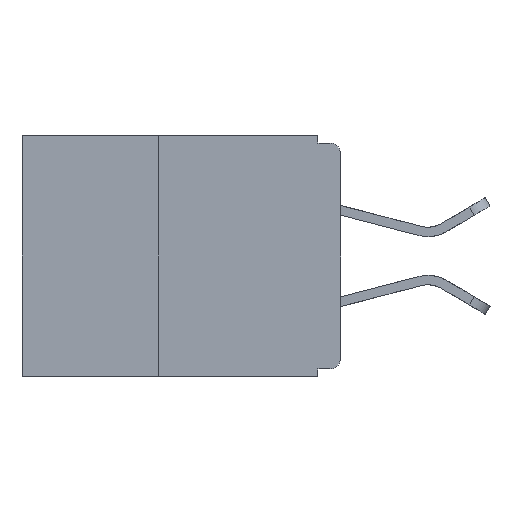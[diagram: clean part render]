
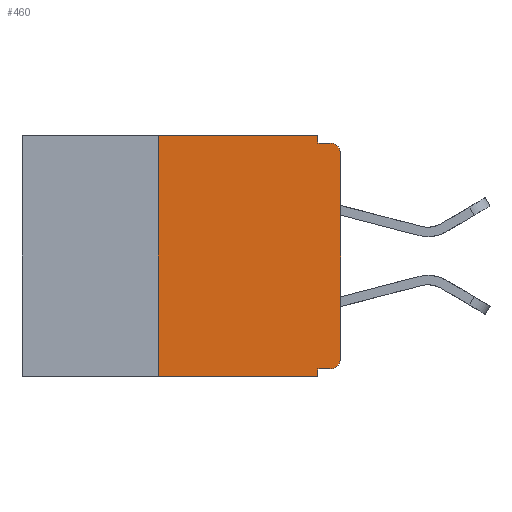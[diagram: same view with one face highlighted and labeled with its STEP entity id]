
A CAD part, left-side view. The second image highlights one B-rep face of the part: STEP entity #460.
In plain terms, the highlighted planar face has unit normal (-1, 0, 0).
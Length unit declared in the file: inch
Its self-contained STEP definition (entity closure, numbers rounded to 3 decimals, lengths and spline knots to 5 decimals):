
#223 = DIRECTION ( 'NONE',  ( 0., 0., -1. ) ) ;
#285 = EDGE_CURVE ( 'NONE', #17375, #4428, #4743, .T. ) ;
#400 = EDGE_CURVE ( 'NONE', #8476, #15993, #18680, .T. ) ;
#460 = ADVANCED_FACE ( 'NONE', ( #1088 ), #10878, .F. ) ;
#977 = CARTESIAN_POINT ( 'NONE',  ( 0., 0.031, 0. ) ) ;
#1088 = FACE_OUTER_BOUND ( 'NONE', #18383, .T. ) ;
#1360 = ORIENTED_EDGE ( 'NONE', *, *, #400, .F. ) ;
#1376 = ORIENTED_EDGE ( 'NONE', *, *, #17903, .F. ) ;
#2164 = CARTESIAN_POINT ( 'NONE',  ( 0., 0.015, -0.01 ) ) ;
#2228 = CARTESIAN_POINT ( 'NONE',  ( 0., 0., 0. ) ) ;
#2318 = DIRECTION ( 'NONE',  ( 0., -1., 0. ) ) ;
#2415 = CARTESIAN_POINT ( 'NONE',  ( 0., 0.437, 0. ) ) ;
#2435 = VERTEX_POINT ( 'NONE', #8285 ) ;
#3471 = AXIS2_PLACEMENT_3D ( 'NONE', #15699, #6561, #17208 ) ;
#3631 = CIRCLE ( 'NONE', #3471, 0.015 ) ;
#3760 = DIRECTION ( 'NONE',  ( 0., 0., -1. ) ) ;
#4344 = VECTOR ( 'NONE', #7113, 39.37008 ) ;
#4399 = LINE ( 'NONE', #14602, #10470 ) ;
#4428 = VERTEX_POINT ( 'NONE', #18686 ) ;
#4743 = LINE ( 'NONE', #12650, #12577 ) ;
#5002 = ORIENTED_EDGE ( 'NONE', *, *, #285, .F. ) ;
#6561 = DIRECTION ( 'NONE',  ( -1., 0., 0. ) ) ;
#6858 = AXIS2_PLACEMENT_3D ( 'NONE', #18980, #9917, #223 ) ;
#7113 = DIRECTION ( 'NONE',  ( 0., 1., 0. ) ) ;
#7298 = VECTOR ( 'NONE', #2318, 39.37008 ) ;
#7758 = VERTEX_POINT ( 'NONE', #977 ) ;
#7860 = CARTESIAN_POINT ( 'NONE',  ( 0., 0.25, 0. ) ) ;
#7988 = LINE ( 'NONE', #19134, #11572 ) ;
#8125 = LINE ( 'NONE', #2228, #15703 ) ;
#8285 = CARTESIAN_POINT ( 'NONE',  ( 0., 0., -0.305 ) ) ;
#8476 = VERTEX_POINT ( 'NONE', #13540 ) ;
#8479 = ORIENTED_EDGE ( 'NONE', *, *, #14955, .F. ) ;
#8782 = EDGE_CURVE ( 'NONE', #18211, #7758, #19862, .T. ) ;
#9809 = CARTESIAN_POINT ( 'NONE',  ( 0., 0.25, -0.33 ) ) ;
#9901 = ORIENTED_EDGE ( 'NONE', *, *, #8782, .F. ) ;
#9917 = DIRECTION ( 'NONE',  ( -1., 0., 0. ) ) ;
#10164 = CARTESIAN_POINT ( 'NONE',  ( 0., 0.25, -0.33 ) ) ;
#10266 = DIRECTION ( 'NONE',  ( 0., 0., 1. ) ) ;
#10390 = EDGE_CURVE ( 'NONE', #17261, #18211, #15106, .T. ) ;
#10470 = VECTOR ( 'NONE', #19138, 39.37008 ) ;
#10646 = VECTOR ( 'NONE', #19593, 39.37008 ) ;
#10878 = PLANE ( 'NONE',  #16770 ) ;
#11572 = VECTOR ( 'NONE', #3760, 39.37008 ) ;
#11605 = ORIENTED_EDGE ( 'NONE', *, *, #17921, .T. ) ;
#11906 = CARTESIAN_POINT ( 'NONE',  ( 0., 0.437, 0. ) ) ;
#12577 = VECTOR ( 'NONE', #15708, 39.37008 ) ;
#12650 = CARTESIAN_POINT ( 'NONE',  ( 0., 0.031, -0.33 ) ) ;
#12839 = EDGE_CURVE ( 'NONE', #15668, #2435, #18295, .T. ) ;
#13505 = CARTESIAN_POINT ( 'NONE',  ( 0., 0.031, -0.32 ) ) ;
#13540 = CARTESIAN_POINT ( 'NONE',  ( 0., 0.031, -0.01 ) ) ;
#14484 = DIRECTION ( 'NONE',  ( 1., 0., 0. ) ) ;
#14602 = CARTESIAN_POINT ( 'NONE',  ( 0., 0.437, -0.33 ) ) ;
#14638 = VECTOR ( 'NONE', #18871, 39.37008 ) ;
#14902 = DIRECTION ( 'NONE',  ( 0., 0., -1. ) ) ;
#14955 = EDGE_CURVE ( 'NONE', #7758, #8476, #7988, .T. ) ;
#15106 = LINE ( 'NONE', #9809, #14638 ) ;
#15367 = ORIENTED_EDGE ( 'NONE', *, *, #15965, .T. ) ;
#15597 = ORIENTED_EDGE ( 'NONE', *, *, #10390, .F. ) ;
#15668 = VERTEX_POINT ( 'NONE', #18117 ) ;
#15699 = CARTESIAN_POINT ( 'NONE',  ( 0., 0.015, -0.025 ) ) ;
#15703 = VECTOR ( 'NONE', #10266, 39.37008 ) ;
#15708 = DIRECTION ( 'NONE',  ( 0., 0., -1. ) ) ;
#15795 = EDGE_CURVE ( 'NONE', #18207, #15993, #3631, .T. ) ;
#15965 = EDGE_CURVE ( 'NONE', #17261, #4428, #4399, .T. ) ;
#15993 = VERTEX_POINT ( 'NONE', #2164 ) ;
#16525 = ORIENTED_EDGE ( 'NONE', *, *, #15795, .T. ) ;
#16770 = AXIS2_PLACEMENT_3D ( 'NONE', #11906, #14484, #14902 ) ;
#16918 = CARTESIAN_POINT ( 'NONE',  ( 0., 0., -0.025 ) ) ;
#17208 = DIRECTION ( 'NONE',  ( 0., 0., -1. ) ) ;
#17261 = VERTEX_POINT ( 'NONE', #10164 ) ;
#17375 = VERTEX_POINT ( 'NONE', #13505 ) ;
#17903 = EDGE_CURVE ( 'NONE', #15668, #17375, #20160, .T. ) ;
#17921 = EDGE_CURVE ( 'NONE', #2435, #18207, #8125, .T. ) ;
#18117 = CARTESIAN_POINT ( 'NONE',  ( 0., 0.015, -0.32 ) ) ;
#18207 = VERTEX_POINT ( 'NONE', #16918 ) ;
#18211 = VERTEX_POINT ( 'NONE', #7860 ) ;
#18295 = CIRCLE ( 'NONE', #6858, 0.015 ) ;
#18299 = CARTESIAN_POINT ( 'NONE',  ( 0., 0., -0.01 ) ) ;
#18383 = EDGE_LOOP ( 'NONE', ( #11605, #16525, #1360, #8479, #9901, #15597, #15367, #5002, #1376, #18735 ) ) ;
#18680 = LINE ( 'NONE', #18299, #10646 ) ;
#18686 = CARTESIAN_POINT ( 'NONE',  ( 0., 0.031, -0.33 ) ) ;
#18735 = ORIENTED_EDGE ( 'NONE', *, *, #12839, .T. ) ;
#18871 = DIRECTION ( 'NONE',  ( 0., 0., 1. ) ) ;
#18980 = CARTESIAN_POINT ( 'NONE',  ( 0., 0.015, -0.305 ) ) ;
#19134 = CARTESIAN_POINT ( 'NONE',  ( 0., 0.031, 0. ) ) ;
#19138 = DIRECTION ( 'NONE',  ( 0., -1., 0. ) ) ;
#19269 = CARTESIAN_POINT ( 'NONE',  ( 0., 0., -0.32 ) ) ;
#19593 = DIRECTION ( 'NONE',  ( 0., -1., 0. ) ) ;
#19862 = LINE ( 'NONE', #2415, #7298 ) ;
#20160 = LINE ( 'NONE', #19269, #4344 ) ;
